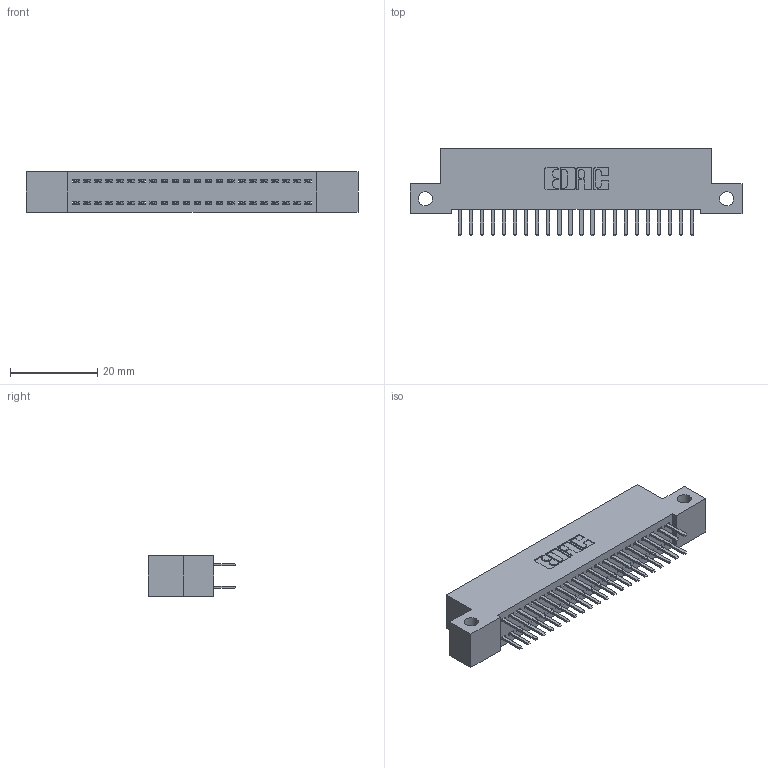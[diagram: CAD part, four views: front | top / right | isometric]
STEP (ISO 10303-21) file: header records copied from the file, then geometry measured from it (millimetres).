
FILE_DESCRIPTION (( 'STEP AP203' ), '1' );
FILE_NAME ('342-044-520-212.STEP', '2019-10-02T18:55:40', ( '' ), ( '' ), 'SwSTEP 2.0', 'SolidWorks 2016', '' );
FILE_SCHEMA (( 'CONFIG_CONTROL_DESIGN' ));
Length unit declared in the file: inch
Products named in the file (3): 342 Part_Side Mount; 345-292-001_345-293-120; 342-044-520-212
Assembly tree (45 placements, depth 2):
  342-044-520-212
    342 Part_Side Mount
    345-292-001_345-293-120  x44
Bounding box: 76.2 x 20.02 x 9.4 mm (x, y, z)
Volume: 6658.6 mm3; surface area: 10140.4 mm2
Topology: 45 solids, 45 shells, 2574 faces, 7471 edges, 4862 vertices
Faces by surface type: plane 1738, cylinder 836
Entity records: 16725 total; most frequent: CARTESIAN_POINT 2806, ORIENTED_EDGE 2730, DIRECTION 2421, EDGE_CURVE 1365, VECTOR 1233, LINE 1233, VERTEX_POINT 906, AXIS2_PLACEMENT_3D 594
